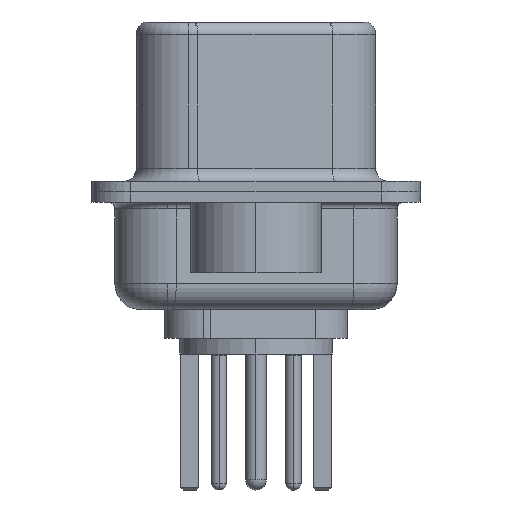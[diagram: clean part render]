
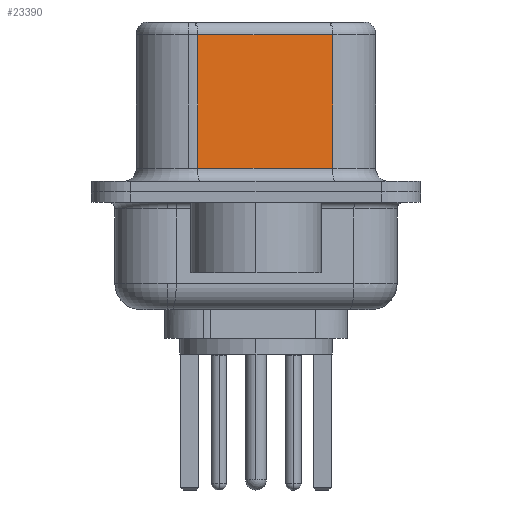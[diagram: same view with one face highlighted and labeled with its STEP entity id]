
A CAD part, left-side view. The second image highlights one B-rep face of the part: STEP entity #23390.
In plain terms, the highlighted planar face has unit normal (-0.985, -0.174, 0).
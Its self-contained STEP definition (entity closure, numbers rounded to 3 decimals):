
#787 = CARTESIAN_POINT ( 'NONE',  ( 3.67, 2.233, 6.02 ) ) ;
#1603 = EDGE_CURVE ( 'NONE', #9281, #13206, #9969, .T. ) ;
#2759 = EDGE_LOOP ( 'NONE', ( #12492, #17666, #21319, #8941 ) ) ;
#2816 = VECTOR ( 'NONE', #20566, 1000. ) ;
#3743 = EDGE_CURVE ( 'NONE', #6819, #13206, #14003, .T. ) ;
#3983 = DIRECTION ( 'NONE',  ( 0.985, 0.174, 0. ) ) ;
#4692 = CARTESIAN_POINT ( 'NONE',  ( 3.67, 2.233, 6.52 ) ) ;
#6580 = DIRECTION ( 'NONE',  ( 0., 0., -1. ) ) ;
#6819 = VERTEX_POINT ( 'NONE', #8948 ) ;
#8205 = LINE ( 'NONE', #4692, #17646 ) ;
#8457 = EDGE_CURVE ( 'NONE', #6819, #16456, #23053, .T. ) ;
#8941 = ORIENTED_EDGE ( 'NONE', *, *, #1603, .T. ) ;
#8948 = CARTESIAN_POINT ( 'NONE',  ( 4.58, -2.927, 6.02 ) ) ;
#9281 = VERTEX_POINT ( 'NONE', #21109 ) ;
#9585 = AXIS2_PLACEMENT_3D ( 'NONE', #20918, #3983, #17155 ) ;
#9969 = LINE ( 'NONE', #19824, #23904 ) ;
#12492 = ORIENTED_EDGE ( 'NONE', *, *, #3743, .F. ) ;
#12892 = EDGE_CURVE ( 'NONE', #16456, #9281, #8205, .T. ) ;
#13206 = VERTEX_POINT ( 'NONE', #16601 ) ;
#13594 = DIRECTION ( 'NONE',  ( 0.174, -0.985, 0. ) ) ;
#14003 = LINE ( 'NONE', #24413, #2816 ) ;
#16456 = VERTEX_POINT ( 'NONE', #787 ) ;
#16601 = CARTESIAN_POINT ( 'NONE',  ( 4.58, -2.927, 0.9 ) ) ;
#16779 = VECTOR ( 'NONE', #16962, 1000. ) ;
#16962 = DIRECTION ( 'NONE',  ( -0.174, 0.985, 0. ) ) ;
#17155 = DIRECTION ( 'NONE',  ( -0.174, 0.985, 0. ) ) ;
#17646 = VECTOR ( 'NONE', #6580, 1000. ) ;
#17666 = ORIENTED_EDGE ( 'NONE', *, *, #8457, .T. ) ;
#19824 = CARTESIAN_POINT ( 'NONE',  ( 4.58, -2.927, 0.9 ) ) ;
#20566 = DIRECTION ( 'NONE',  ( 0., 0., -1. ) ) ;
#20918 = CARTESIAN_POINT ( 'NONE',  ( 4.58, -2.927, 6.52 ) ) ;
#21109 = CARTESIAN_POINT ( 'NONE',  ( 3.67, 2.233, 0.9 ) ) ;
#21319 = ORIENTED_EDGE ( 'NONE', *, *, #12892, .T. ) ;
#22844 = PLANE ( 'NONE',  #9585 ) ;
#23053 = LINE ( 'NONE', #24320, #16779 ) ;
#23390 = ADVANCED_FACE ( 'NONE', ( #24247 ), #22844, .F. ) ;
#23904 = VECTOR ( 'NONE', #13594, 1000. ) ;
#24247 = FACE_OUTER_BOUND ( 'NONE', #2759, .T. ) ;
#24320 = CARTESIAN_POINT ( 'NONE',  ( 4.58, -2.927, 6.02 ) ) ;
#24413 = CARTESIAN_POINT ( 'NONE',  ( 4.58, -2.927, 6.52 ) ) ;
